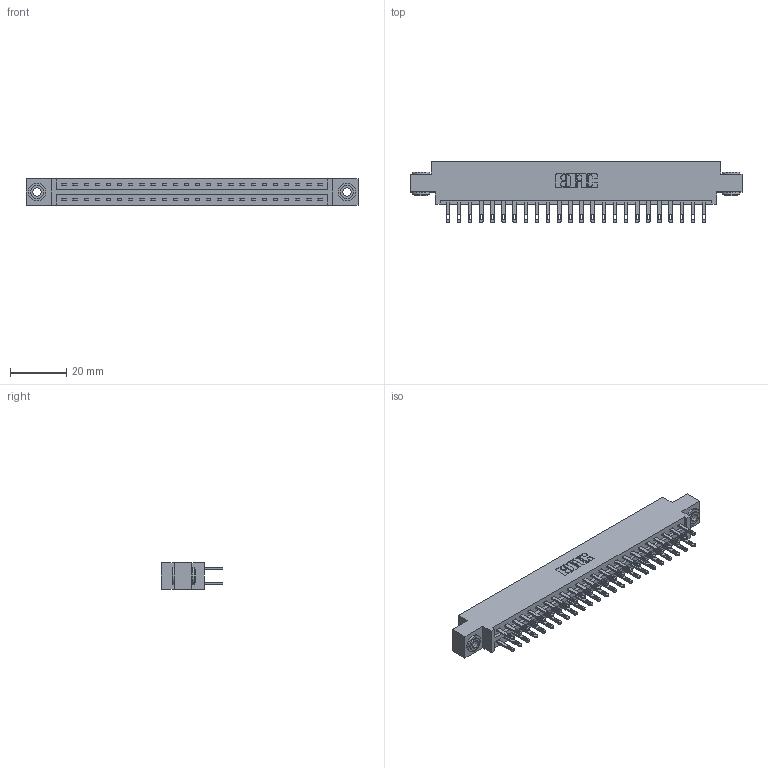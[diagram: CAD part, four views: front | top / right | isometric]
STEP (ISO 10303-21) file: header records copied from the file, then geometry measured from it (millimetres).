
FILE_DESCRIPTION (( 'STEP AP203' ), '1' );
FILE_NAME ('887-048-500-803.STEP', '2020-09-21T00:56:56', ( '' ), ( '' ), 'SwSTEP 2.0', 'SolidWorks 2020', '' );
FILE_SCHEMA (( 'CONFIG_CONTROL_DESIGN' ));
Length unit declared in the file: inch
Products named in the file (4): 345-250-002_345-250-002-102; 887-048-500-803; 837 Part_0.170 Offset - 0.156 Dia-TH; 345-292-001_345-293-100
Assembly tree (51 placements, depth 2):
  887-048-500-803
    837 Part_0.170 Offset - 0.156 Dia-TH
    345-292-001_345-293-100  x48
    345-250-002_345-250-002-102  x2
Bounding box: 118.11 x 21.85 x 9.4 mm (x, y, z)
Volume: 12256.3 mm3; surface area: 14545.8 mm2
Topology: 51 solids, 51 shells, 2556 faces, 7743 edges, 5158 vertices
Faces by surface type: plane 1620, cylinder 928, cone 8
Entity records: 21648 total; most frequent: CARTESIAN_POINT 3637, ORIENTED_EDGE 3566, DIRECTION 3161, EDGE_CURVE 1783, LINE 1627, VECTOR 1627, VERTEX_POINT 1186, AXIS2_PLACEMENT_3D 767
